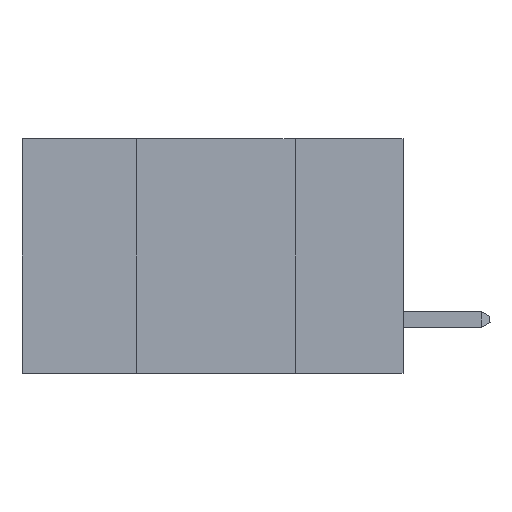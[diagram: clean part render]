
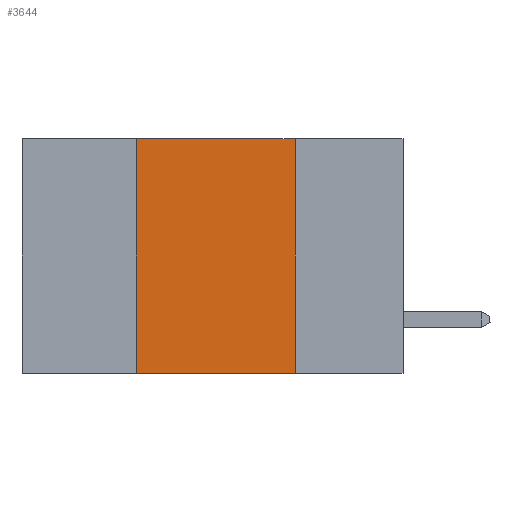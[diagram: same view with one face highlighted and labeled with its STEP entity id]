
A CAD part, left-side view. The second image highlights one B-rep face of the part: STEP entity #3644.
In plain terms, the highlighted planar face has unit normal (-1, 0, 0).
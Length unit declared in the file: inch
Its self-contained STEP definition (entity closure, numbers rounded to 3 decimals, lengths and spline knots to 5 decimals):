
#1163 = DIRECTION ( 'NONE',  ( 0., 0., -1. ) ) ;
#1207 = VECTOR ( 'NONE', #16169, 39.37008 ) ;
#1337 = CARTESIAN_POINT ( 'NONE',  ( 0., 0.17, 0. ) ) ;
#1783 = LINE ( 'NONE', #9565, #13186 ) ;
#1796 = ORIENTED_EDGE ( 'NONE', *, *, #24735, .F. ) ;
#1953 = CARTESIAN_POINT ( 'NONE',  ( 0., 0.6, -0.37 ) ) ;
#3644 = ADVANCED_FACE ( 'NONE', ( #9973 ), #5264, .F. ) ;
#5092 = DIRECTION ( 'NONE',  ( 1., 0., 0. ) ) ;
#5237 = CARTESIAN_POINT ( 'NONE',  ( 0., 0.42, -0.37 ) ) ;
#5264 = PLANE ( 'NONE',  #24301 ) ;
#5487 = VERTEX_POINT ( 'NONE', #23680 ) ;
#6476 = EDGE_CURVE ( 'NONE', #17766, #21641, #9566, .T. ) ;
#7390 = DIRECTION ( 'NONE',  ( 0., 0., -1. ) ) ;
#7827 = CARTESIAN_POINT ( 'NONE',  ( 0., 0.42, 0. ) ) ;
#7984 = EDGE_LOOP ( 'NONE', ( #1796, #23826, #10099, #25500 ) ) ;
#9267 = VECTOR ( 'NONE', #10145, 39.37008 ) ;
#9565 = CARTESIAN_POINT ( 'NONE',  ( 0., 0.17, 0. ) ) ;
#9566 = LINE ( 'NONE', #1953, #1207 ) ;
#9973 = FACE_OUTER_BOUND ( 'NONE', #7984, .T. ) ;
#10077 = LINE ( 'NONE', #10984, #24863 ) ;
#10099 = ORIENTED_EDGE ( 'NONE', *, *, #21318, .F. ) ;
#10145 = DIRECTION ( 'NONE',  ( 0., 0., 1. ) ) ;
#10188 = VERTEX_POINT ( 'NONE', #1337 ) ;
#10984 = CARTESIAN_POINT ( 'NONE',  ( 0., 0.6, 0. ) ) ;
#11072 = DIRECTION ( 'NONE',  ( 0., -1., 0. ) ) ;
#13186 = VECTOR ( 'NONE', #7390, 39.37008 ) ;
#16169 = DIRECTION ( 'NONE',  ( 0., -1., 0. ) ) ;
#17766 = VERTEX_POINT ( 'NONE', #5237 ) ;
#21318 = EDGE_CURVE ( 'NONE', #17766, #5487, #24670, .T. ) ;
#21641 = VERTEX_POINT ( 'NONE', #24781 ) ;
#23338 = EDGE_CURVE ( 'NONE', #5487, #10188, #10077, .T. ) ;
#23680 = CARTESIAN_POINT ( 'NONE',  ( 0., 0.42, 0. ) ) ;
#23826 = ORIENTED_EDGE ( 'NONE', *, *, #23338, .F. ) ;
#24301 = AXIS2_PLACEMENT_3D ( 'NONE', #24827, #5092, #1163 ) ;
#24670 = LINE ( 'NONE', #7827, #9267 ) ;
#24735 = EDGE_CURVE ( 'NONE', #10188, #21641, #1783, .T. ) ;
#24781 = CARTESIAN_POINT ( 'NONE',  ( 0., 0.17, -0.37 ) ) ;
#24827 = CARTESIAN_POINT ( 'NONE',  ( 0., 0.6, 0. ) ) ;
#24863 = VECTOR ( 'NONE', #11072, 39.37008 ) ;
#25500 = ORIENTED_EDGE ( 'NONE', *, *, #6476, .T. ) ;
